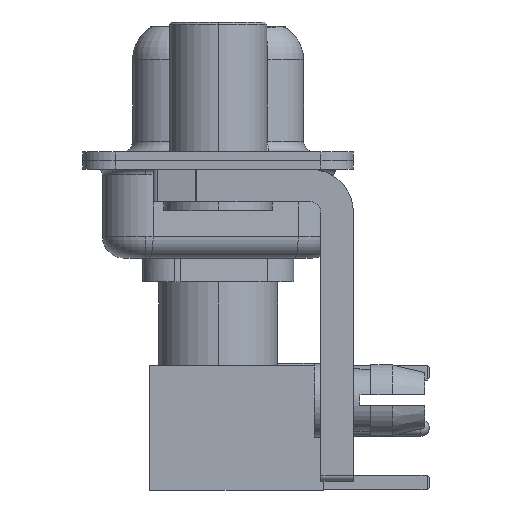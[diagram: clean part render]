
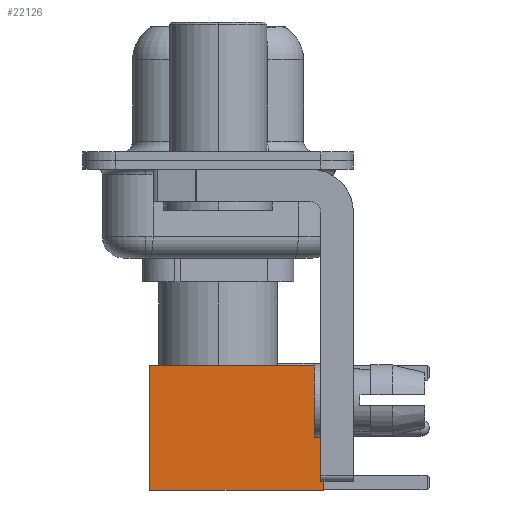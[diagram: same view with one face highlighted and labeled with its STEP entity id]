
A CAD part, left-side view. The second image highlights one B-rep face of the part: STEP entity #22126.
In plain terms, the highlighted face is planar.
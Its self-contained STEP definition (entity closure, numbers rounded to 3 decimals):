
#499 = ORIENTED_EDGE ( 'NONE', *, *, #20412, .T. ) ;
#609 = DIRECTION ( 'NONE',  ( -1., 0., 0. ) ) ;
#762 = CARTESIAN_POINT ( 'NONE',  ( 2.875, 2.875, 0. ) ) ;
#917 = EDGE_CURVE ( 'NONE', #3761, #21481, #9747, .T. ) ;
#1262 = VERTEX_POINT ( 'NONE', #19144 ) ;
#1456 = LINE ( 'NONE', #18819, #8078 ) ;
#2362 = VECTOR ( 'NONE', #10676, 1000. ) ;
#3761 = VERTEX_POINT ( 'NONE', #23812 ) ;
#3797 = DIRECTION ( 'NONE',  ( 0., 1., 0. ) ) ;
#4621 = EDGE_CURVE ( 'NONE', #22975, #1262, #7309, .T. ) ;
#6180 = PLANE ( 'NONE',  #22018 ) ;
#6526 = VECTOR ( 'NONE', #22649, 1000. ) ;
#7309 = LINE ( 'NONE', #22141, #2362 ) ;
#7870 = DIRECTION ( 'NONE',  ( 0., 0., 1. ) ) ;
#8078 = VECTOR ( 'NONE', #9150, 1000. ) ;
#9150 = DIRECTION ( 'NONE',  ( -1., 0., 0. ) ) ;
#9467 = ORIENTED_EDGE ( 'NONE', *, *, #9875, .F. ) ;
#9588 = ORIENTED_EDGE ( 'NONE', *, *, #917, .F. ) ;
#9747 = LINE ( 'NONE', #15284, #6526 ) ;
#9875 = EDGE_CURVE ( 'NONE', #22975, #3761, #13374, .T. ) ;
#10046 = EDGE_LOOP ( 'NONE', ( #13569, #499, #9588, #9467 ) ) ;
#10676 = DIRECTION ( 'NONE',  ( 0., 0., -1. ) ) ;
#11138 = FACE_OUTER_BOUND ( 'NONE', #10046, .T. ) ;
#12505 = CARTESIAN_POINT ( 'NONE',  ( 2.875, 2.875, 8. ) ) ;
#13374 = LINE ( 'NONE', #18461, #22904 ) ;
#13569 = ORIENTED_EDGE ( 'NONE', *, *, #4621, .T. ) ;
#15284 = CARTESIAN_POINT ( 'NONE',  ( -2.875, 2.875, 0. ) ) ;
#18461 = CARTESIAN_POINT ( 'NONE',  ( 0., 2.875, 8. ) ) ;
#18819 = CARTESIAN_POINT ( 'NONE',  ( 0., 2.875, 0. ) ) ;
#18850 = CARTESIAN_POINT ( 'NONE',  ( -2.875, 2.875, 0. ) ) ;
#19144 = CARTESIAN_POINT ( 'NONE',  ( 2.875, 2.875, 0. ) ) ;
#20412 = EDGE_CURVE ( 'NONE', #1262, #21481, #1456, .T. ) ;
#21481 = VERTEX_POINT ( 'NONE', #18850 ) ;
#22018 = AXIS2_PLACEMENT_3D ( 'NONE', #762, #3797, #7870 ) ;
#22126 = ADVANCED_FACE ( 'NONE', ( #11138 ), #6180, .T. ) ;
#22141 = CARTESIAN_POINT ( 'NONE',  ( 2.875, 2.875, 0. ) ) ;
#22649 = DIRECTION ( 'NONE',  ( 0., 0., -1. ) ) ;
#22904 = VECTOR ( 'NONE', #609, 1000. ) ;
#22975 = VERTEX_POINT ( 'NONE', #12505 ) ;
#23812 = CARTESIAN_POINT ( 'NONE',  ( -2.875, 2.875, 8. ) ) ;
